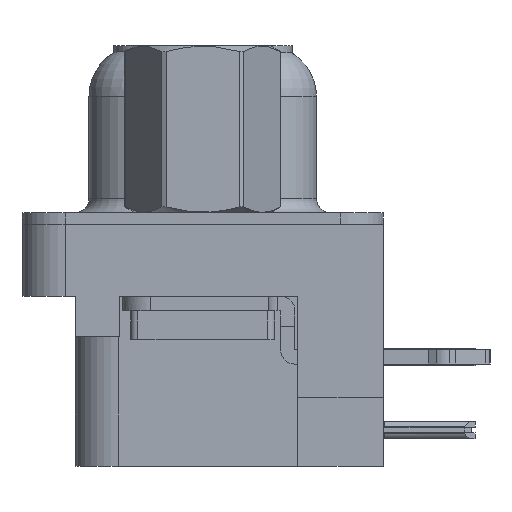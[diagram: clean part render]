
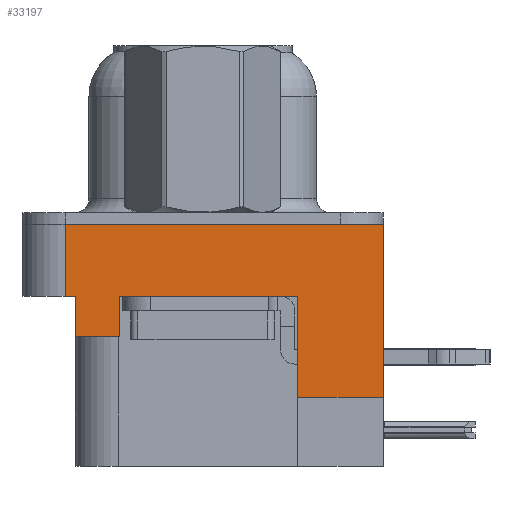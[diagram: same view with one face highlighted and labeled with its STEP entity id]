
A CAD part, left-side view. The second image highlights one B-rep face of the part: STEP entity #33197.
In plain terms, the highlighted planar face has unit normal (-1, 0, 0).
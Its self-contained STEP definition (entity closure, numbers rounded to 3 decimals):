
#53 = ORIENTED_EDGE ( 'NONE', *, *, #9416, .F. ) ;
#583 = VERTEX_POINT ( 'NONE', #22229 ) ;
#1003 = EDGE_CURVE ( 'NONE', #7807, #20791, #32089, .T. ) ;
#1209 = EDGE_CURVE ( 'NONE', #7221, #2280, #12227, .T. ) ;
#1332 = CARTESIAN_POINT ( 'NONE',  ( -3., 4.775, -2.5 ) ) ;
#1389 = PLANE ( 'NONE',  #9347 ) ;
#1561 = DIRECTION ( 'NONE',  ( 0., 0., 1. ) ) ;
#2280 = VERTEX_POINT ( 'NONE', #29201 ) ;
#2332 = VECTOR ( 'NONE', #33199, 1000. ) ;
#3846 = DIRECTION ( 'NONE',  ( 0., 0., 1. ) ) ;
#4312 = VECTOR ( 'NONE', #28133, 1000. ) ;
#5047 = VERTEX_POINT ( 'NONE', #21534 ) ;
#5074 = CARTESIAN_POINT ( 'NONE',  ( -3., 4.425, -3.9 ) ) ;
#5335 = LINE ( 'NONE', #25891, #19142 ) ;
#5910 = VECTOR ( 'NONE', #24762, 1000. ) ;
#6872 = DIRECTION ( 'NONE',  ( -1., 0., 0. ) ) ;
#7221 = VERTEX_POINT ( 'NONE', #31651 ) ;
#7365 = CARTESIAN_POINT ( 'NONE',  ( -3., -3.295, -8.4 ) ) ;
#7807 = VERTEX_POINT ( 'NONE', #21094 ) ;
#7900 = CARTESIAN_POINT ( 'NONE',  ( -3., -3.295, -2.5 ) ) ;
#8022 = DIRECTION ( 'NONE',  ( 0., 1., 0. ) ) ;
#8378 = CARTESIAN_POINT ( 'NONE',  ( -3., -6.275, -2.5 ) ) ;
#9347 = AXIS2_PLACEMENT_3D ( 'NONE', #17827, #6872, #26171 ) ;
#9416 = EDGE_CURVE ( 'NONE', #20791, #5047, #28669, .T. ) ;
#9585 = ORIENTED_EDGE ( 'NONE', *, *, #1003, .F. ) ;
#9679 = EDGE_CURVE ( 'NONE', #7221, #5047, #23455, .T. ) ;
#9880 = LINE ( 'NONE', #11937, #4312 ) ;
#10070 = VECTOR ( 'NONE', #21175, 1000. ) ;
#10204 = CARTESIAN_POINT ( 'NONE',  ( -3., -6.275, -2.5 ) ) ;
#10558 = ORIENTED_EDGE ( 'NONE', *, *, #23108, .F. ) ;
#10784 = VECTOR ( 'NONE', #8022, 1000. ) ;
#11937 = CARTESIAN_POINT ( 'NONE',  ( -3., -6.275, 0. ) ) ;
#12227 = LINE ( 'NONE', #1332, #33358 ) ;
#12703 = ORIENTED_EDGE ( 'NONE', *, *, #9679, .T. ) ;
#13238 = LINE ( 'NONE', #21955, #5910 ) ;
#13452 = CARTESIAN_POINT ( 'NONE',  ( -3., -6.495, -6. ) ) ;
#13892 = VECTOR ( 'NONE', #18415, 1000. ) ;
#14874 = CARTESIAN_POINT ( 'NONE',  ( -3., 2.895, -2.5 ) ) ;
#16106 = VECTOR ( 'NONE', #21183, 1000. ) ;
#16712 = DIRECTION ( 'NONE',  ( 0., 0., 1. ) ) ;
#16926 = LINE ( 'NONE', #8378, #2332 ) ;
#17013 = EDGE_LOOP ( 'NONE', ( #24915, #35291, #10558, #25559, #12703, #53, #9585, #29359, #31105, #20053 ) ) ;
#17827 = CARTESIAN_POINT ( 'NONE',  ( -3., -6.275, -2.5 ) ) ;
#18136 = LINE ( 'NONE', #13452, #10784 ) ;
#18415 = DIRECTION ( 'NONE',  ( 0., 0., 1. ) ) ;
#18454 = CARTESIAN_POINT ( 'NONE',  ( -3., -3.295, -6. ) ) ;
#19142 = VECTOR ( 'NONE', #3846, 1000. ) ;
#20053 = ORIENTED_EDGE ( 'NONE', *, *, #21200, .F. ) ;
#20419 = CARTESIAN_POINT ( 'NONE',  ( -3., 4.425, -3.9 ) ) ;
#20791 = VERTEX_POINT ( 'NONE', #5074 ) ;
#21094 = CARTESIAN_POINT ( 'NONE',  ( -3., 2.895, -3.9 ) ) ;
#21175 = DIRECTION ( 'NONE',  ( 0., 1., 0. ) ) ;
#21183 = DIRECTION ( 'NONE',  ( 0., -1., 0. ) ) ;
#21200 = EDGE_CURVE ( 'NONE', #30033, #31260, #28565, .T. ) ;
#21534 = CARTESIAN_POINT ( 'NONE',  ( -3., 4.425, -2.5 ) ) ;
#21955 = CARTESIAN_POINT ( 'NONE',  ( -3., -6.275, -2.5 ) ) ;
#22229 = CARTESIAN_POINT ( 'NONE',  ( -3., -6.275, 0. ) ) ;
#23108 = EDGE_CURVE ( 'NONE', #2280, #583, #9880, .T. ) ;
#23295 = VERTEX_POINT ( 'NONE', #23750 ) ;
#23455 = LINE ( 'NONE', #10204, #16106 ) ;
#23750 = CARTESIAN_POINT ( 'NONE',  ( -3., -6.275, -6. ) ) ;
#24011 = EDGE_CURVE ( 'NONE', #23295, #30033, #18136, .T. ) ;
#24762 = DIRECTION ( 'NONE',  ( 0., -1., 0. ) ) ;
#24915 = ORIENTED_EDGE ( 'NONE', *, *, #24011, .F. ) ;
#25559 = ORIENTED_EDGE ( 'NONE', *, *, #1209, .F. ) ;
#25891 = CARTESIAN_POINT ( 'NONE',  ( -3., 2.895, -3.9 ) ) ;
#26171 = DIRECTION ( 'NONE',  ( 0., 0., 1. ) ) ;
#27039 = EDGE_CURVE ( 'NONE', #31684, #31260, #13238, .T. ) ;
#27753 = CARTESIAN_POINT ( 'NONE',  ( -3., 4.425, -3.9 ) ) ;
#28133 = DIRECTION ( 'NONE',  ( 0., -1., 0. ) ) ;
#28565 = LINE ( 'NONE', #7365, #13892 ) ;
#28669 = LINE ( 'NONE', #27753, #35079 ) ;
#29201 = CARTESIAN_POINT ( 'NONE',  ( -3., 4.775, 0. ) ) ;
#29333 = EDGE_CURVE ( 'NONE', #7807, #31684, #5335, .T. ) ;
#29359 = ORIENTED_EDGE ( 'NONE', *, *, #29333, .T. ) ;
#29717 = FACE_OUTER_BOUND ( 'NONE', #17013, .T. ) ;
#30033 = VERTEX_POINT ( 'NONE', #18454 ) ;
#31105 = ORIENTED_EDGE ( 'NONE', *, *, #27039, .T. ) ;
#31260 = VERTEX_POINT ( 'NONE', #7900 ) ;
#31405 = EDGE_CURVE ( 'NONE', #23295, #583, #16926, .T. ) ;
#31651 = CARTESIAN_POINT ( 'NONE',  ( -3., 4.775, -2.5 ) ) ;
#31684 = VERTEX_POINT ( 'NONE', #14874 ) ;
#32089 = LINE ( 'NONE', #20419, #10070 ) ;
#33197 = ADVANCED_FACE ( 'NONE', ( #29717 ), #1389, .T. ) ;
#33199 = DIRECTION ( 'NONE',  ( 0., 0., 1. ) ) ;
#33358 = VECTOR ( 'NONE', #1561, 1000. ) ;
#35079 = VECTOR ( 'NONE', #16712, 1000. ) ;
#35291 = ORIENTED_EDGE ( 'NONE', *, *, #31405, .T. ) ;
